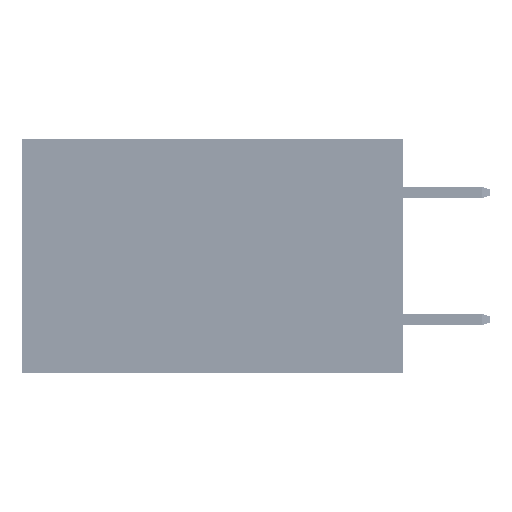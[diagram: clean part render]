
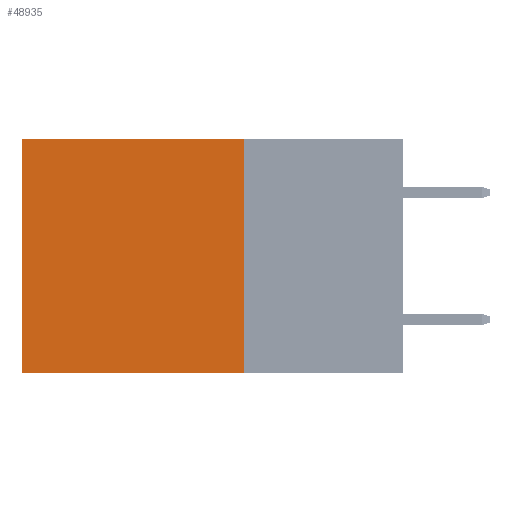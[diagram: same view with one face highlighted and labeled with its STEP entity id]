
A CAD part, left-side view. The second image highlights one B-rep face of the part: STEP entity #48935.
In plain terms, the highlighted planar face has unit normal (-1, 0, 0).
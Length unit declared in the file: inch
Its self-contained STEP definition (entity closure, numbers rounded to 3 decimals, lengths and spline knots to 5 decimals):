
#560 = EDGE_CURVE ( 'NONE', #39246, #3721, #7743, .T. ) ;
#592 = LINE ( 'NONE', #19469, #5692 ) ;
#2248 = EDGE_LOOP ( 'NONE', ( #46402, #45545, #6440, #23572 ) ) ;
#3721 = VERTEX_POINT ( 'NONE', #45809 ) ;
#5692 = VECTOR ( 'NONE', #11776, 39.37008 ) ;
#6126 = CARTESIAN_POINT ( 'NONE',  ( 0.2875, 0.25, 0. ) ) ;
#6440 = ORIENTED_EDGE ( 'NONE', *, *, #560, .F. ) ;
#6824 = DIRECTION ( 'NONE',  ( 0., 0., -1. ) ) ;
#7743 = LINE ( 'NONE', #37612, #39032 ) ;
#11006 = VERTEX_POINT ( 'NONE', #13362 ) ;
#11776 = DIRECTION ( 'NONE',  ( 0., 1., 0. ) ) ;
#13362 = CARTESIAN_POINT ( 'NONE',  ( 0.2875, 0.6, 0. ) ) ;
#14223 = PLANE ( 'NONE',  #31459 ) ;
#14903 = DIRECTION ( 'NONE',  ( 0., 0., -1. ) ) ;
#15224 = EDGE_CURVE ( 'NONE', #39246, #11006, #25032, .T. ) ;
#19469 = CARTESIAN_POINT ( 'NONE',  ( 0.2875, 0.25, -0.37 ) ) ;
#23572 = ORIENTED_EDGE ( 'NONE', *, *, #15224, .T. ) ;
#24011 = VECTOR ( 'NONE', #25733, 39.37008 ) ;
#24770 = DIRECTION ( 'NONE',  ( 0., 1., 0. ) ) ;
#25032 = LINE ( 'NONE', #6126, #38490 ) ;
#25733 = DIRECTION ( 'NONE',  ( 0., 0., -1. ) ) ;
#31459 = AXIS2_PLACEMENT_3D ( 'NONE', #48416, #32955, #6824 ) ;
#32955 = DIRECTION ( 'NONE',  ( 1., 0., 0. ) ) ;
#33196 = FACE_OUTER_BOUND ( 'NONE', #2248, .T. ) ;
#33207 = LINE ( 'NONE', #48426, #24011 ) ;
#37612 = CARTESIAN_POINT ( 'NONE',  ( 0.2875, 0.25, 0. ) ) ;
#37802 = EDGE_CURVE ( 'NONE', #3721, #45452, #592, .T. ) ;
#37987 = CARTESIAN_POINT ( 'NONE',  ( 0.2875, 0.6, -0.37 ) ) ;
#38389 = EDGE_CURVE ( 'NONE', #11006, #45452, #33207, .T. ) ;
#38490 = VECTOR ( 'NONE', #24770, 39.37008 ) ;
#39032 = VECTOR ( 'NONE', #14903, 39.37008 ) ;
#39246 = VERTEX_POINT ( 'NONE', #45247 ) ;
#45247 = CARTESIAN_POINT ( 'NONE',  ( 0.2875, 0.25, 0. ) ) ;
#45452 = VERTEX_POINT ( 'NONE', #37987 ) ;
#45545 = ORIENTED_EDGE ( 'NONE', *, *, #37802, .F. ) ;
#45809 = CARTESIAN_POINT ( 'NONE',  ( 0.2875, 0.25, -0.37 ) ) ;
#46402 = ORIENTED_EDGE ( 'NONE', *, *, #38389, .T. ) ;
#48416 = CARTESIAN_POINT ( 'NONE',  ( 0.2875, 0.25, 0. ) ) ;
#48426 = CARTESIAN_POINT ( 'NONE',  ( 0.2875, 0.6, 0. ) ) ;
#48935 = ADVANCED_FACE ( 'NONE', ( #33196 ), #14223, .F. ) ;
